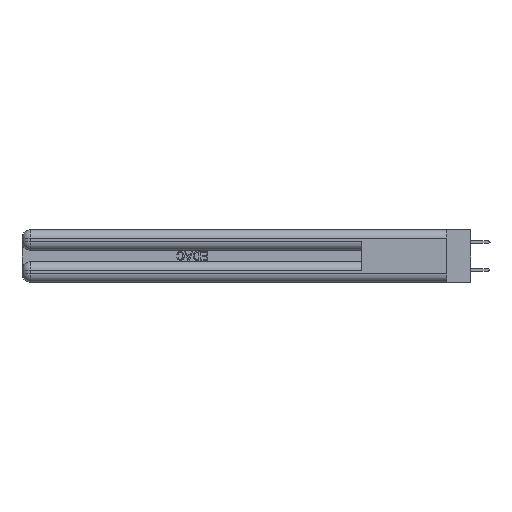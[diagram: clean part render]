
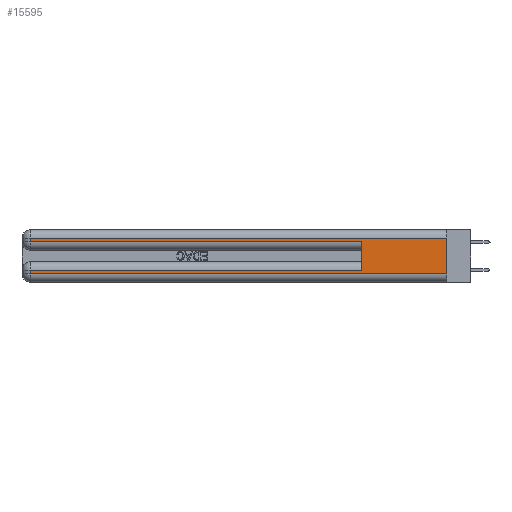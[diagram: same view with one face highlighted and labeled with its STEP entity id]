
A CAD part, left-side view. The second image highlights one B-rep face of the part: STEP entity #15595.
In plain terms, the highlighted planar face has unit normal (-1, 0, 0).
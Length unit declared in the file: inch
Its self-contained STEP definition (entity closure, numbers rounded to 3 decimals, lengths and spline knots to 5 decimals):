
#158 = LINE ( 'NONE', #16352, #19314 ) ;
#379 = ORIENTED_EDGE ( 'NONE', *, *, #21535, .F. ) ;
#570 = VECTOR ( 'NONE', #22927, 39.37008 ) ;
#1673 = LINE ( 'NONE', #23996, #2742 ) ;
#1883 = DIRECTION ( 'NONE',  ( 0., 0., -1. ) ) ;
#2742 = VECTOR ( 'NONE', #20818, 39.37008 ) ;
#2751 = EDGE_LOOP ( 'NONE', ( #379, #14579, #5398, #18846, #21013, #30680, #34427, #7539 ) ) ;
#4047 = VERTEX_POINT ( 'NONE', #22090 ) ;
#5139 = LINE ( 'NONE', #18380, #21655 ) ;
#5207 = CARTESIAN_POINT ( 'NONE',  ( 0., 0., 0.31 ) ) ;
#5398 = ORIENTED_EDGE ( 'NONE', *, *, #31719, .T. ) ;
#7513 = CARTESIAN_POINT ( 'NONE',  ( 0., 0.6, 0.085 ) ) ;
#7539 = ORIENTED_EDGE ( 'NONE', *, *, #38469, .T. ) ;
#7763 = LINE ( 'NONE', #30323, #16930 ) ;
#8443 = VERTEX_POINT ( 'NONE', #40084 ) ;
#11132 = CARTESIAN_POINT ( 'NONE',  ( 0., 0., 0.37 ) ) ;
#11828 = CARTESIAN_POINT ( 'NONE',  ( 0., 0., 0.06 ) ) ;
#12521 = CARTESIAN_POINT ( 'NONE',  ( 0., 0., 0.37 ) ) ;
#12722 = DIRECTION ( 'NONE',  ( 0., 0., -1. ) ) ;
#12900 = EDGE_CURVE ( 'NONE', #17963, #34472, #22706, .T. ) ;
#13693 = VECTOR ( 'NONE', #12722, 39.37008 ) ;
#14065 = DIRECTION ( 'NONE',  ( 1., 0., 0. ) ) ;
#14352 = EDGE_CURVE ( 'NONE', #19415, #4047, #1673, .T. ) ;
#14579 = ORIENTED_EDGE ( 'NONE', *, *, #30585, .T. ) ;
#14986 = LINE ( 'NONE', #11828, #26346 ) ;
#15464 = CARTESIAN_POINT ( 'NONE',  ( 0., 2.94, 0.285 ) ) ;
#15595 = ADVANCED_FACE ( 'NONE', ( #30331 ), #40015, .F. ) ;
#15885 = LINE ( 'NONE', #12521, #13693 ) ;
#16008 = VERTEX_POINT ( 'NONE', #7513 ) ;
#16352 = CARTESIAN_POINT ( 'NONE',  ( 0., 2.94, 0.37 ) ) ;
#16930 = VECTOR ( 'NONE', #26944, 39.37008 ) ;
#17963 = VERTEX_POINT ( 'NONE', #15464 ) ;
#18380 = CARTESIAN_POINT ( 'NONE',  ( 0., 0.6, 0.145 ) ) ;
#18456 = EDGE_CURVE ( 'NONE', #16008, #34472, #5139, .T. ) ;
#18846 = ORIENTED_EDGE ( 'NONE', *, *, #12900, .T. ) ;
#19314 = VECTOR ( 'NONE', #28628, 39.37008 ) ;
#19415 = VERTEX_POINT ( 'NONE', #27267 ) ;
#20818 = DIRECTION ( 'NONE',  ( 0., 0., -1. ) ) ;
#21013 = ORIENTED_EDGE ( 'NONE', *, *, #18456, .F. ) ;
#21535 = EDGE_CURVE ( 'NONE', #31956, #8443, #15885, .T. ) ;
#21655 = VECTOR ( 'NONE', #21959, 39.37008 ) ;
#21959 = DIRECTION ( 'NONE',  ( 0., 0., 1. ) ) ;
#22090 = CARTESIAN_POINT ( 'NONE',  ( 0., 2.94, 0.06 ) ) ;
#22706 = LINE ( 'NONE', #35597, #570 ) ;
#22927 = DIRECTION ( 'NONE',  ( 0., -1., 0. ) ) ;
#23107 = CARTESIAN_POINT ( 'NONE',  ( 0., 0., 0.31 ) ) ;
#23996 = CARTESIAN_POINT ( 'NONE',  ( 0., 2.94, 0.37 ) ) ;
#25130 = DIRECTION ( 'NONE',  ( 0., -1., 0. ) ) ;
#26346 = VECTOR ( 'NONE', #25130, 39.37008 ) ;
#26688 = DIRECTION ( 'NONE',  ( 0., 1., 0. ) ) ;
#26944 = DIRECTION ( 'NONE',  ( 0., 1., 0. ) ) ;
#27267 = CARTESIAN_POINT ( 'NONE',  ( 0., 2.94, 0.085 ) ) ;
#28628 = DIRECTION ( 'NONE',  ( 0., 0., -1. ) ) ;
#28765 = VERTEX_POINT ( 'NONE', #41083 ) ;
#30323 = CARTESIAN_POINT ( 'NONE',  ( 0., 0., 0.085 ) ) ;
#30331 = FACE_OUTER_BOUND ( 'NONE', #2751, .T. ) ;
#30585 = EDGE_CURVE ( 'NONE', #31956, #28765, #33021, .T. ) ;
#30680 = ORIENTED_EDGE ( 'NONE', *, *, #39196, .T. ) ;
#31602 = AXIS2_PLACEMENT_3D ( 'NONE', #11132, #14065, #1883 ) ;
#31719 = EDGE_CURVE ( 'NONE', #28765, #17963, #158, .T. ) ;
#31956 = VERTEX_POINT ( 'NONE', #5207 ) ;
#33021 = LINE ( 'NONE', #23107, #40128 ) ;
#34427 = ORIENTED_EDGE ( 'NONE', *, *, #14352, .T. ) ;
#34472 = VERTEX_POINT ( 'NONE', #38678 ) ;
#35597 = CARTESIAN_POINT ( 'NONE',  ( 0., 0., 0.285 ) ) ;
#38469 = EDGE_CURVE ( 'NONE', #4047, #8443, #14986, .T. ) ;
#38678 = CARTESIAN_POINT ( 'NONE',  ( 0., 0.6, 0.285 ) ) ;
#39196 = EDGE_CURVE ( 'NONE', #16008, #19415, #7763, .T. ) ;
#40015 = PLANE ( 'NONE',  #31602 ) ;
#40084 = CARTESIAN_POINT ( 'NONE',  ( 0., 0., 0.06 ) ) ;
#40128 = VECTOR ( 'NONE', #26688, 39.37008 ) ;
#41083 = CARTESIAN_POINT ( 'NONE',  ( 0., 2.94, 0.31 ) ) ;
